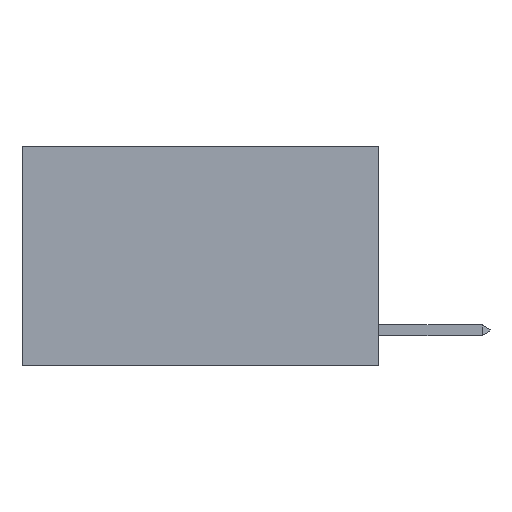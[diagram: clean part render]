
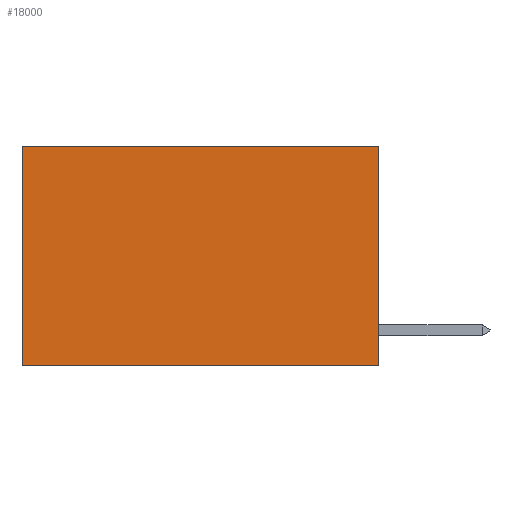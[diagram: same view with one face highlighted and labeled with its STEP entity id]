
A CAD part, left-side view. The second image highlights one B-rep face of the part: STEP entity #18000.
In plain terms, the highlighted planar face has unit normal (-1, 0, 0).
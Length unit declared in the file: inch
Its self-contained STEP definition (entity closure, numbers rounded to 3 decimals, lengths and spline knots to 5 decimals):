
#307 = DIRECTION ( 'NONE',  ( 0., 1., 0. ) ) ;
#1415 = FACE_OUTER_BOUND ( 'NONE', #7856, .T. ) ;
#1443 = CARTESIAN_POINT ( 'NONE',  ( 0.2625, 0., 0. ) ) ;
#1958 = LINE ( 'NONE', #8757, #14643 ) ;
#2115 = VERTEX_POINT ( 'NONE', #1443 ) ;
#2687 = VERTEX_POINT ( 'NONE', #3746 ) ;
#2810 = ORIENTED_EDGE ( 'NONE', *, *, #11869, .T. ) ;
#3544 = PLANE ( 'NONE',  #8235 ) ;
#3746 = CARTESIAN_POINT ( 'NONE',  ( 0.2625, 0.6, 0. ) ) ;
#5412 = ORIENTED_EDGE ( 'NONE', *, *, #13177, .T. ) ;
#7731 = EDGE_CURVE ( 'NONE', #2115, #8120, #10457, .T. ) ;
#7856 = EDGE_LOOP ( 'NONE', ( #5412, #19671, #19859, #2810 ) ) ;
#8120 = VERTEX_POINT ( 'NONE', #10684 ) ;
#8235 = AXIS2_PLACEMENT_3D ( 'NONE', #16750, #8956, #14795 ) ;
#8757 = CARTESIAN_POINT ( 'NONE',  ( 0.2625, 0., 0. ) ) ;
#8796 = EDGE_CURVE ( 'NONE', #8120, #20960, #9425, .T. ) ;
#8956 = DIRECTION ( 'NONE',  ( 1., 0., 0. ) ) ;
#9425 = LINE ( 'NONE', #13346, #14784 ) ;
#10457 = LINE ( 'NONE', #20160, #10726 ) ;
#10684 = CARTESIAN_POINT ( 'NONE',  ( 0.2625, 0., -0.37 ) ) ;
#10726 = VECTOR ( 'NONE', #14465, 39.37008 ) ;
#11869 = EDGE_CURVE ( 'NONE', #2115, #2687, #1958, .T. ) ;
#13177 = EDGE_CURVE ( 'NONE', #2687, #20960, #16905, .T. ) ;
#13346 = CARTESIAN_POINT ( 'NONE',  ( 0.2625, 0., -0.37 ) ) ;
#13528 = DIRECTION ( 'NONE',  ( 0., 0., -1. ) ) ;
#14465 = DIRECTION ( 'NONE',  ( 0., 0., -1. ) ) ;
#14643 = VECTOR ( 'NONE', #20208, 39.37008 ) ;
#14784 = VECTOR ( 'NONE', #307, 39.37008 ) ;
#14795 = DIRECTION ( 'NONE',  ( 0., 0., -1. ) ) ;
#16750 = CARTESIAN_POINT ( 'NONE',  ( 0.2625, 0., 0. ) ) ;
#16905 = LINE ( 'NONE', #17215, #23402 ) ;
#17215 = CARTESIAN_POINT ( 'NONE',  ( 0.2625, 0.6, 0. ) ) ;
#18000 = ADVANCED_FACE ( 'NONE', ( #1415 ), #3544, .F. ) ;
#19671 = ORIENTED_EDGE ( 'NONE', *, *, #8796, .F. ) ;
#19859 = ORIENTED_EDGE ( 'NONE', *, *, #7731, .F. ) ;
#20160 = CARTESIAN_POINT ( 'NONE',  ( 0.2625, 0., 0. ) ) ;
#20208 = DIRECTION ( 'NONE',  ( 0., 1., 0. ) ) ;
#20960 = VERTEX_POINT ( 'NONE', #23807 ) ;
#23402 = VECTOR ( 'NONE', #13528, 39.37008 ) ;
#23807 = CARTESIAN_POINT ( 'NONE',  ( 0.2625, 0.6, -0.37 ) ) ;
